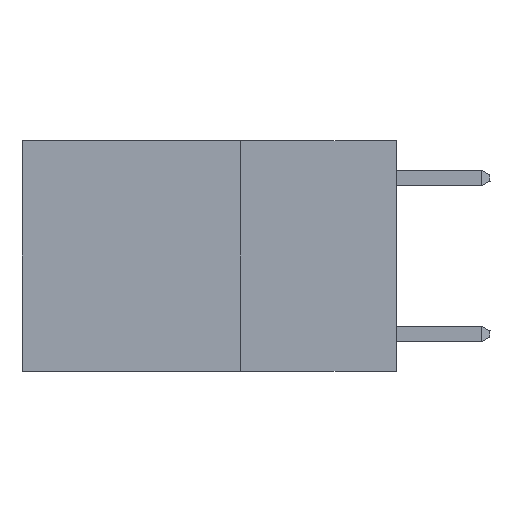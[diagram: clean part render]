
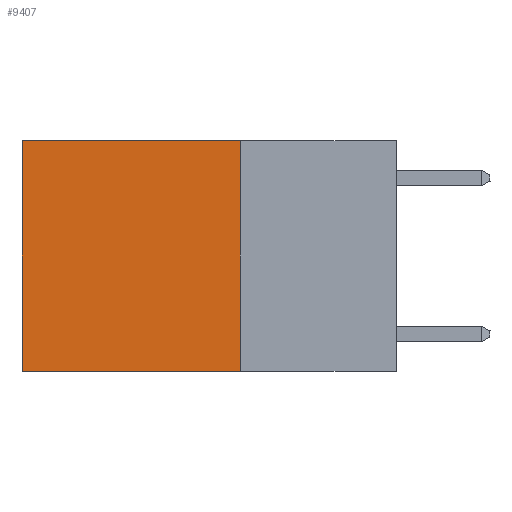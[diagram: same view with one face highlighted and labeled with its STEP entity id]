
A CAD part, left-side view. The second image highlights one B-rep face of the part: STEP entity #9407.
In plain terms, the highlighted planar face has unit normal (-1, 0, 0).
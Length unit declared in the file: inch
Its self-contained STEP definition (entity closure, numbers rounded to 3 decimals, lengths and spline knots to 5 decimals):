
#263 = ORIENTED_EDGE ( 'NONE', *, *, #3904, .F. ) ;
#532 = EDGE_CURVE ( 'NONE', #743, #5128, #8509, .T. ) ;
#655 = VERTEX_POINT ( 'NONE', #4792 ) ;
#743 = VERTEX_POINT ( 'NONE', #8880 ) ;
#759 = DIRECTION ( 'NONE',  ( 1., 0., 0. ) ) ;
#874 = EDGE_CURVE ( 'NONE', #4104, #655, #3785, .T. ) ;
#1221 = CARTESIAN_POINT ( 'NONE',  ( 0.2625, 0.6, 0. ) ) ;
#1281 = DIRECTION ( 'NONE',  ( 0., 0., -1. ) ) ;
#1417 = ORIENTED_EDGE ( 'NONE', *, *, #5070, .T. ) ;
#1997 = AXIS2_PLACEMENT_3D ( 'NONE', #5292, #759, #5359 ) ;
#2016 = CARTESIAN_POINT ( 'NONE',  ( 0.2625, 0.25, 0. ) ) ;
#2752 = DIRECTION ( 'NONE',  ( 0., 1., 0. ) ) ;
#3487 = CARTESIAN_POINT ( 'NONE',  ( 0.2625, 0.25, -0.37 ) ) ;
#3785 = LINE ( 'NONE', #3487, #8504 ) ;
#3904 = EDGE_CURVE ( 'NONE', #743, #4104, #5953, .T. ) ;
#3954 = VECTOR ( 'NONE', #1281, 39.37008 ) ;
#4104 = VERTEX_POINT ( 'NONE', #8368 ) ;
#4250 = VECTOR ( 'NONE', #4319, 39.37008 ) ;
#4319 = DIRECTION ( 'NONE',  ( 0., 0., -1. ) ) ;
#4379 = DIRECTION ( 'NONE',  ( 0., 1., 0. ) ) ;
#4487 = LINE ( 'NONE', #8854, #4250 ) ;
#4600 = VECTOR ( 'NONE', #4379, 39.37008 ) ;
#4792 = CARTESIAN_POINT ( 'NONE',  ( 0.2625, 0.6, -0.37 ) ) ;
#5070 = EDGE_CURVE ( 'NONE', #5128, #655, #4487, .T. ) ;
#5128 = VERTEX_POINT ( 'NONE', #1221 ) ;
#5292 = CARTESIAN_POINT ( 'NONE',  ( 0.2625, 0.25, 0. ) ) ;
#5359 = DIRECTION ( 'NONE',  ( 0., 0., -1. ) ) ;
#5515 = ORIENTED_EDGE ( 'NONE', *, *, #874, .F. ) ;
#5804 = ORIENTED_EDGE ( 'NONE', *, *, #532, .T. ) ;
#5953 = LINE ( 'NONE', #2016, #3954 ) ;
#6816 = EDGE_LOOP ( 'NONE', ( #1417, #5515, #263, #5804 ) ) ;
#7380 = CARTESIAN_POINT ( 'NONE',  ( 0.2625, 0.25, 0. ) ) ;
#7630 = PLANE ( 'NONE',  #1997 ) ;
#8368 = CARTESIAN_POINT ( 'NONE',  ( 0.2625, 0.25, -0.37 ) ) ;
#8504 = VECTOR ( 'NONE', #2752, 39.37008 ) ;
#8509 = LINE ( 'NONE', #7380, #4600 ) ;
#8854 = CARTESIAN_POINT ( 'NONE',  ( 0.2625, 0.6, 0. ) ) ;
#8880 = CARTESIAN_POINT ( 'NONE',  ( 0.2625, 0.25, 0. ) ) ;
#9215 = FACE_OUTER_BOUND ( 'NONE', #6816, .T. ) ;
#9407 = ADVANCED_FACE ( 'NONE', ( #9215 ), #7630, .F. ) ;
